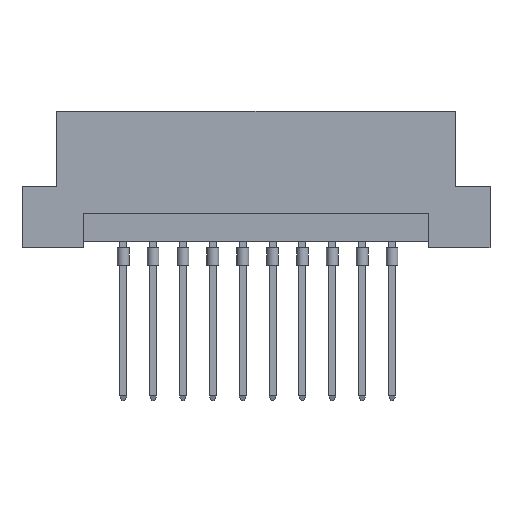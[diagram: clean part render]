
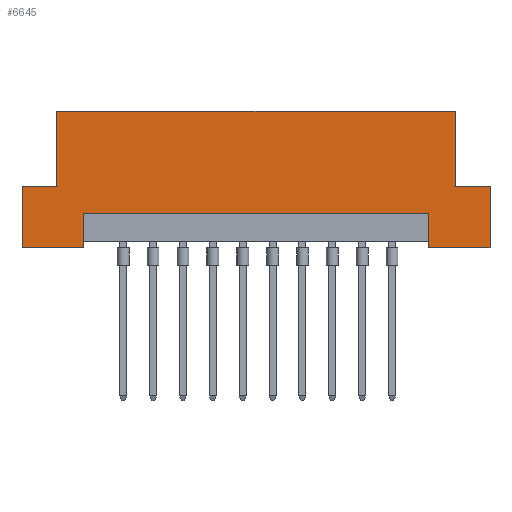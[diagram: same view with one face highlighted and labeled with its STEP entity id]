
A CAD part, front view. The second image highlights one B-rep face of the part: STEP entity #6645.
In plain terms, the highlighted planar face has unit normal (0, -1, 0).
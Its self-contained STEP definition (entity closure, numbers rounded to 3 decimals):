
#38 = LINE ( 'NONE', #1157, #857 ) ;
#111 = CARTESIAN_POINT ( 'NONE',  ( 16.94, 0., 5.2 ) ) ;
#271 = VECTOR ( 'NONE', #750, 1000. ) ;
#293 = CARTESIAN_POINT ( 'NONE',  ( 14.69, 0., 0.5 ) ) ;
#317 = ORIENTED_EDGE ( 'NONE', *, *, #6327, .F. ) ;
#322 = CARTESIAN_POINT ( 'NONE',  ( -14.69, 0., 0.5 ) ) ;
#341 = ORIENTED_EDGE ( 'NONE', *, *, #2549, .T. ) ;
#388 = CARTESIAN_POINT ( 'NONE',  ( -14.69, 0., 2.9 ) ) ;
#437 = EDGE_CURVE ( 'NONE', #3215, #5903, #5243, .T. ) ;
#438 = DIRECTION ( 'NONE',  ( 0., 0., 1. ) ) ;
#480 = LINE ( 'NONE', #1607, #6336 ) ;
#528 = ORIENTED_EDGE ( 'NONE', *, *, #838, .F. ) ;
#657 = LINE ( 'NONE', #111, #5760 ) ;
#749 = EDGE_LOOP ( 'NONE', ( #6013, #6852, #6099, #1224, #1038, #341, #317, #5617, #3135, #528, #5107, #4934 ) ) ;
#750 = DIRECTION ( 'NONE',  ( -1., 0., 0. ) ) ;
#774 = CARTESIAN_POINT ( 'NONE',  ( -19.9, 0., 5.2 ) ) ;
#813 = VERTEX_POINT ( 'NONE', #5563 ) ;
#838 = EDGE_CURVE ( 'NONE', #3061, #6875, #480, .T. ) ;
#857 = VECTOR ( 'NONE', #4551, 1000. ) ;
#939 = CARTESIAN_POINT ( 'NONE',  ( -14.69, 0., 0. ) ) ;
#979 = DIRECTION ( 'NONE',  ( 0., 1., 0. ) ) ;
#997 = LINE ( 'NONE', #3233, #1529 ) ;
#1038 = ORIENTED_EDGE ( 'NONE', *, *, #4313, .F. ) ;
#1157 = CARTESIAN_POINT ( 'NONE',  ( -19.9, 0., 0. ) ) ;
#1224 = ORIENTED_EDGE ( 'NONE', *, *, #2511, .F. ) ;
#1267 = DIRECTION ( 'NONE',  ( 0., 0., -1. ) ) ;
#1529 = VECTOR ( 'NONE', #5468, 1000. ) ;
#1556 = VECTOR ( 'NONE', #1267, 1000. ) ;
#1593 = CARTESIAN_POINT ( 'NONE',  ( 19.9, 0., 5.2 ) ) ;
#1607 = CARTESIAN_POINT ( 'NONE',  ( -19.9, 0., 0. ) ) ;
#1979 = DIRECTION ( 'NONE',  ( 0., 0., -1. ) ) ;
#1999 = LINE ( 'NONE', #6921, #5949 ) ;
#2012 = DIRECTION ( 'NONE',  ( 0., 0., -1. ) ) ;
#2040 = CARTESIAN_POINT ( 'NONE',  ( 14.69, 0., 2.9 ) ) ;
#2045 = LINE ( 'NONE', #6340, #2368 ) ;
#2137 = AXIS2_PLACEMENT_3D ( 'NONE', #6135, #979, #438 ) ;
#2141 = DIRECTION ( 'NONE',  ( 0., 0., 1. ) ) ;
#2196 = CARTESIAN_POINT ( 'NONE',  ( 14.69, 0., 0. ) ) ;
#2368 = VECTOR ( 'NONE', #5945, 1000. ) ;
#2417 = EDGE_CURVE ( 'NONE', #2684, #4336, #38, .T. ) ;
#2428 = VERTEX_POINT ( 'NONE', #4514 ) ;
#2436 = DIRECTION ( 'NONE',  ( 1., 0., 0. ) ) ;
#2451 = DIRECTION ( 'NONE',  ( 0., 0., 1. ) ) ;
#2511 = EDGE_CURVE ( 'NONE', #3980, #2684, #4625, .T. ) ;
#2524 = CARTESIAN_POINT ( 'NONE',  ( 19.9, 0., 0. ) ) ;
#2549 = EDGE_CURVE ( 'NONE', #2428, #5120, #657, .T. ) ;
#2684 = VERTEX_POINT ( 'NONE', #2524 ) ;
#2717 = VERTEX_POINT ( 'NONE', #939 ) ;
#3060 = EDGE_CURVE ( 'NONE', #6875, #6712, #1999, .T. ) ;
#3061 = VERTEX_POINT ( 'NONE', #4655 ) ;
#3135 = ORIENTED_EDGE ( 'NONE', *, *, #3060, .F. ) ;
#3215 = VERTEX_POINT ( 'NONE', #2040 ) ;
#3233 = CARTESIAN_POINT ( 'NONE',  ( -19.9, 0., 0. ) ) ;
#3348 = EDGE_CURVE ( 'NONE', #2717, #3061, #997, .T. ) ;
#3353 = DIRECTION ( 'NONE',  ( 1., 0., 0. ) ) ;
#3466 = CARTESIAN_POINT ( 'NONE',  ( 19.9, 0., 5.2 ) ) ;
#3591 = CARTESIAN_POINT ( 'NONE',  ( -19.9, 0., 11.6 ) ) ;
#3642 = EDGE_CURVE ( 'NONE', #3215, #4336, #5882, .T. ) ;
#3868 = VECTOR ( 'NONE', #1979, 1000. ) ;
#3916 = FACE_OUTER_BOUND ( 'NONE', #749, .T. ) ;
#3980 = VERTEX_POINT ( 'NONE', #3466 ) ;
#4141 = EDGE_CURVE ( 'NONE', #5903, #2717, #6890, .T. ) ;
#4313 = EDGE_CURVE ( 'NONE', #2428, #3980, #7166, .T. ) ;
#4336 = VERTEX_POINT ( 'NONE', #2196 ) ;
#4514 = CARTESIAN_POINT ( 'NONE',  ( 16.94, 0., 5.2 ) ) ;
#4551 = DIRECTION ( 'NONE',  ( -1., 0., 0. ) ) ;
#4625 = LINE ( 'NONE', #6277, #1556 ) ;
#4646 = CARTESIAN_POINT ( 'NONE',  ( 14.69, 0., 2.9 ) ) ;
#4655 = CARTESIAN_POINT ( 'NONE',  ( -19.9, 0., 0. ) ) ;
#4843 = CARTESIAN_POINT ( 'NONE',  ( 16.94, 0., 11.6 ) ) ;
#4934 = ORIENTED_EDGE ( 'NONE', *, *, #4141, .F. ) ;
#5107 = ORIENTED_EDGE ( 'NONE', *, *, #3348, .F. ) ;
#5120 = VERTEX_POINT ( 'NONE', #4843 ) ;
#5243 = LINE ( 'NONE', #4646, #271 ) ;
#5280 = LINE ( 'NONE', #3591, #6426 ) ;
#5468 = DIRECTION ( 'NONE',  ( -1., 0., 0. ) ) ;
#5563 = CARTESIAN_POINT ( 'NONE',  ( -16.94, 0., 11.6 ) ) ;
#5617 = ORIENTED_EDGE ( 'NONE', *, *, #5869, .F. ) ;
#5760 = VECTOR ( 'NONE', #2451, 1000. ) ;
#5869 = EDGE_CURVE ( 'NONE', #6712, #813, #2045, .T. ) ;
#5882 = LINE ( 'NONE', #293, #3868 ) ;
#5903 = VERTEX_POINT ( 'NONE', #388 ) ;
#5945 = DIRECTION ( 'NONE',  ( 0., 0., 1. ) ) ;
#5949 = VECTOR ( 'NONE', #6335, 1000. ) ;
#5992 = CARTESIAN_POINT ( 'NONE',  ( -16.94, 0., 5.2 ) ) ;
#6013 = ORIENTED_EDGE ( 'NONE', *, *, #437, .F. ) ;
#6099 = ORIENTED_EDGE ( 'NONE', *, *, #2417, .F. ) ;
#6135 = CARTESIAN_POINT ( 'NONE',  ( -19.9, 0., 11.6 ) ) ;
#6146 = PLANE ( 'NONE',  #2137 ) ;
#6277 = CARTESIAN_POINT ( 'NONE',  ( 19.9, 0., 0. ) ) ;
#6327 = EDGE_CURVE ( 'NONE', #813, #5120, #5280, .T. ) ;
#6335 = DIRECTION ( 'NONE',  ( 1., 0., 0. ) ) ;
#6336 = VECTOR ( 'NONE', #2141, 1000. ) ;
#6340 = CARTESIAN_POINT ( 'NONE',  ( -16.94, 0., 5.2 ) ) ;
#6426 = VECTOR ( 'NONE', #2436, 1000. ) ;
#6645 = ADVANCED_FACE ( 'NONE', ( #3916 ), #6146, .F. ) ;
#6693 = VECTOR ( 'NONE', #3353, 1000. ) ;
#6712 = VERTEX_POINT ( 'NONE', #5992 ) ;
#6852 = ORIENTED_EDGE ( 'NONE', *, *, #3642, .T. ) ;
#6875 = VERTEX_POINT ( 'NONE', #774 ) ;
#6890 = LINE ( 'NONE', #322, #7058 ) ;
#6921 = CARTESIAN_POINT ( 'NONE',  ( -19.9, 0., 5.2 ) ) ;
#7058 = VECTOR ( 'NONE', #2012, 1000. ) ;
#7166 = LINE ( 'NONE', #1593, #6693 ) ;
